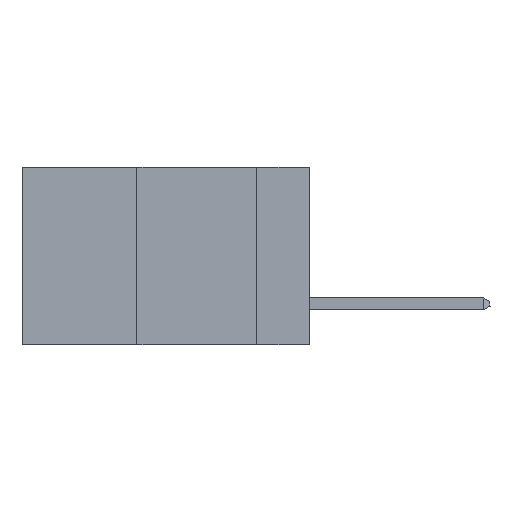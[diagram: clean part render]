
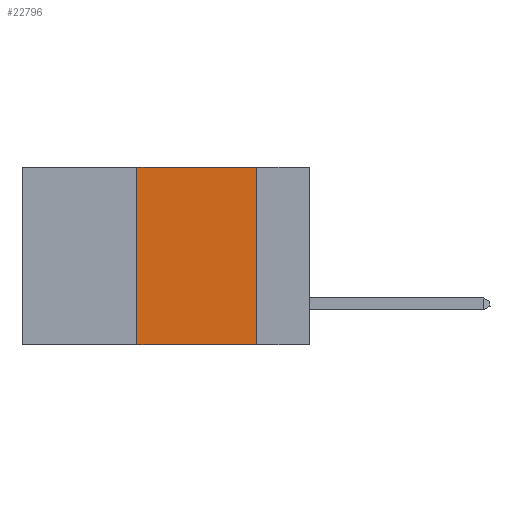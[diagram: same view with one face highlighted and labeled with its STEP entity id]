
A CAD part, left-side view. The second image highlights one B-rep face of the part: STEP entity #22796.
In plain terms, the highlighted planar face has unit normal (-1, 0, 0).
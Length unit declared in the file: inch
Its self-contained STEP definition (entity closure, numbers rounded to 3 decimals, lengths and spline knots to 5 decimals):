
#63 = CARTESIAN_POINT ( 'NONE',  ( 0., 0.6, 0. ) ) ;
#876 = LINE ( 'NONE', #17834, #20078 ) ;
#1370 = LINE ( 'NONE', #11698, #22532 ) ;
#1767 = FACE_OUTER_BOUND ( 'NONE', #22597, .T. ) ;
#2343 = ORIENTED_EDGE ( 'NONE', *, *, #19116, .F. ) ;
#2984 = CARTESIAN_POINT ( 'NONE',  ( 0., 0.11, 0. ) ) ;
#3970 = ORIENTED_EDGE ( 'NONE', *, *, #18876, .F. ) ;
#5296 = LINE ( 'NONE', #12772, #21332 ) ;
#6198 = AXIS2_PLACEMENT_3D ( 'NONE', #63, #18308, #7363 ) ;
#6244 = VECTOR ( 'NONE', #17674, 39.37008 ) ;
#7363 = DIRECTION ( 'NONE',  ( 0., 0., -1. ) ) ;
#7926 = CARTESIAN_POINT ( 'NONE',  ( 0., 0.36, 0. ) ) ;
#10024 = VERTEX_POINT ( 'NONE', #22079 ) ;
#10672 = DIRECTION ( 'NONE',  ( 0., -1., 0. ) ) ;
#11449 = DIRECTION ( 'NONE',  ( 0., 0., 1. ) ) ;
#11698 = CARTESIAN_POINT ( 'NONE',  ( 0., 0.36, 0. ) ) ;
#12772 = CARTESIAN_POINT ( 'NONE',  ( 0., 0.6, 0. ) ) ;
#14291 = DIRECTION ( 'NONE',  ( 0., -1., 0. ) ) ;
#15739 = CARTESIAN_POINT ( 'NONE',  ( 0., 0.11, -0.37 ) ) ;
#16116 = ORIENTED_EDGE ( 'NONE', *, *, #21110, .F. ) ;
#16276 = LINE ( 'NONE', #2984, #6244 ) ;
#16395 = PLANE ( 'NONE',  #6198 ) ;
#17674 = DIRECTION ( 'NONE',  ( 0., 0., -1. ) ) ;
#17834 = CARTESIAN_POINT ( 'NONE',  ( 0., 0.6, -0.37 ) ) ;
#18150 = ORIENTED_EDGE ( 'NONE', *, *, #23354, .T. ) ;
#18308 = DIRECTION ( 'NONE',  ( 1., 0., 0. ) ) ;
#18831 = VERTEX_POINT ( 'NONE', #20164 ) ;
#18876 = EDGE_CURVE ( 'NONE', #10024, #23533, #1370, .T. ) ;
#19116 = EDGE_CURVE ( 'NONE', #18831, #20979, #16276, .T. ) ;
#20078 = VECTOR ( 'NONE', #14291, 39.37008 ) ;
#20164 = CARTESIAN_POINT ( 'NONE',  ( 0., 0.11, 0. ) ) ;
#20979 = VERTEX_POINT ( 'NONE', #15739 ) ;
#21110 = EDGE_CURVE ( 'NONE', #23533, #18831, #5296, .T. ) ;
#21332 = VECTOR ( 'NONE', #10672, 39.37008 ) ;
#22079 = CARTESIAN_POINT ( 'NONE',  ( 0., 0.36, -0.37 ) ) ;
#22532 = VECTOR ( 'NONE', #11449, 39.37008 ) ;
#22597 = EDGE_LOOP ( 'NONE', ( #2343, #16116, #3970, #18150 ) ) ;
#22796 = ADVANCED_FACE ( 'NONE', ( #1767 ), #16395, .F. ) ;
#23354 = EDGE_CURVE ( 'NONE', #10024, #20979, #876, .T. ) ;
#23533 = VERTEX_POINT ( 'NONE', #7926 ) ;
